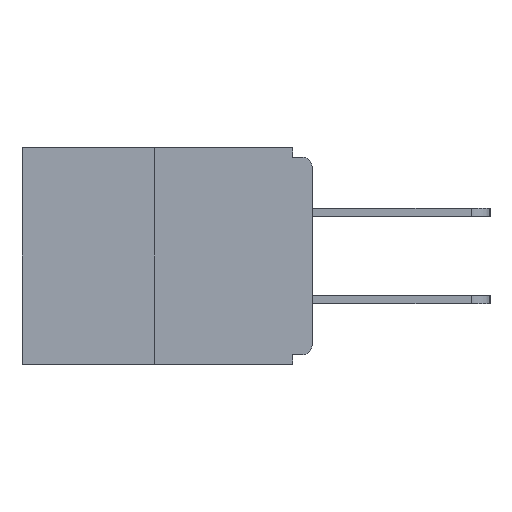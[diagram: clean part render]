
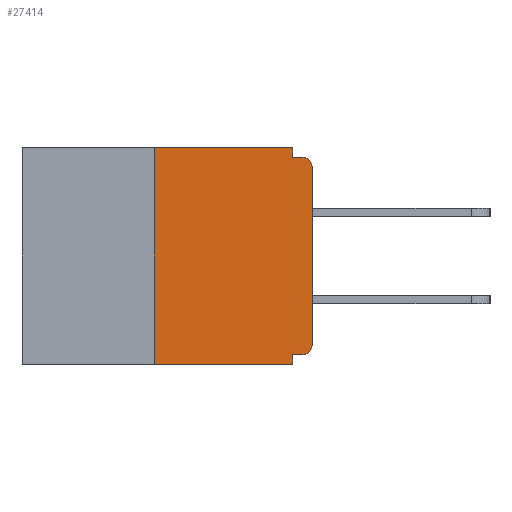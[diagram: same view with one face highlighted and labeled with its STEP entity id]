
A CAD part, left-side view. The second image highlights one B-rep face of the part: STEP entity #27414.
In plain terms, the highlighted planar face has unit normal (-1, 0, 0).
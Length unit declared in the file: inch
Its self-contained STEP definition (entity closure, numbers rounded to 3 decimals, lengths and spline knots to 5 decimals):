
#258 = VERTEX_POINT ( 'NONE', #12342 ) ;
#924 = CIRCLE ( 'NONE', #13292, 0.015 ) ;
#1094 = EDGE_CURVE ( 'NONE', #1641, #19054, #5235, .T. ) ;
#1258 = DIRECTION ( 'NONE',  ( 0., 0., -1. ) ) ;
#1621 = DIRECTION ( 'NONE',  ( 0., 0., -1. ) ) ;
#1641 = VERTEX_POINT ( 'NONE', #3744 ) ;
#2174 = DIRECTION ( 'NONE',  ( -1., 0., 0. ) ) ;
#2730 = CARTESIAN_POINT ( 'NONE',  ( 0., 0., -0.03 ) ) ;
#2752 = CARTESIAN_POINT ( 'NONE',  ( 0., 0.25, 0. ) ) ;
#3408 = ORIENTED_EDGE ( 'NONE', *, *, #23665, .F. ) ;
#3699 = EDGE_CURVE ( 'NONE', #7260, #28635, #924, .T. ) ;
#3744 = CARTESIAN_POINT ( 'NONE',  ( 0., 0.031, 0. ) ) ;
#3880 = ORIENTED_EDGE ( 'NONE', *, *, #10002, .F. ) ;
#4035 = DIRECTION ( 'NONE',  ( -1., 0., 0. ) ) ;
#4437 = VECTOR ( 'NONE', #1258, 39.37008 ) ;
#4613 = ORIENTED_EDGE ( 'NONE', *, *, #25031, .T. ) ;
#4737 = DIRECTION ( 'NONE',  ( 0., -1., 0. ) ) ;
#5190 = ORIENTED_EDGE ( 'NONE', *, *, #6835, .F. ) ;
#5235 = LINE ( 'NONE', #22909, #20057 ) ;
#6483 = CARTESIAN_POINT ( 'NONE',  ( 0., 0., -0.313 ) ) ;
#6586 = CARTESIAN_POINT ( 'NONE',  ( 0., 0., 0. ) ) ;
#6591 = EDGE_CURVE ( 'NONE', #25810, #1641, #14493, .T. ) ;
#6717 = LINE ( 'NONE', #6586, #25359 ) ;
#6772 = CARTESIAN_POINT ( 'NONE',  ( 0., 0., -0.328 ) ) ;
#6835 = EDGE_CURVE ( 'NONE', #19054, #28635, #21328, .T. ) ;
#7096 = VECTOR ( 'NONE', #27136, 39.37008 ) ;
#7260 = VERTEX_POINT ( 'NONE', #2730 ) ;
#8129 = CARTESIAN_POINT ( 'NONE',  ( 0., 0.46, -0.343 ) ) ;
#10002 = EDGE_CURVE ( 'NONE', #25297, #10109, #11707, .T. ) ;
#10061 = ORIENTED_EDGE ( 'NONE', *, *, #30148, .F. ) ;
#10109 = VERTEX_POINT ( 'NONE', #23777 ) ;
#10566 = ORIENTED_EDGE ( 'NONE', *, *, #18706, .T. ) ;
#11361 = VECTOR ( 'NONE', #28966, 39.37008 ) ;
#11636 = CARTESIAN_POINT ( 'NONE',  ( 0., 0.46, 0. ) ) ;
#11707 = LINE ( 'NONE', #18376, #4437 ) ;
#12342 = CARTESIAN_POINT ( 'NONE',  ( 0., 0.25, -0.343 ) ) ;
#13026 = DIRECTION ( 'NONE',  ( 0., -1., 0. ) ) ;
#13292 = AXIS2_PLACEMENT_3D ( 'NONE', #18622, #4035, #18407 ) ;
#13556 = DIRECTION ( 'NONE',  ( 0., 0., -1. ) ) ;
#13570 = LINE ( 'NONE', #2752, #7096 ) ;
#14385 = LINE ( 'NONE', #6772, #11361 ) ;
#14493 = LINE ( 'NONE', #27083, #30835 ) ;
#16056 = CARTESIAN_POINT ( 'NONE',  ( 0., 0.031, -0.328 ) ) ;
#16406 = CARTESIAN_POINT ( 'NONE',  ( 0., 0.25, 0. ) ) ;
#16729 = CARTESIAN_POINT ( 'NONE',  ( 0., 0.015, -0.015 ) ) ;
#17074 = DIRECTION ( 'NONE',  ( 0., -1., 0. ) ) ;
#18250 = EDGE_CURVE ( 'NONE', #18261, #7260, #6717, .T. ) ;
#18261 = VERTEX_POINT ( 'NONE', #6483 ) ;
#18376 = CARTESIAN_POINT ( 'NONE',  ( 0., 0.031, -0.343 ) ) ;
#18407 = DIRECTION ( 'NONE',  ( 0., 0., -1. ) ) ;
#18622 = CARTESIAN_POINT ( 'NONE',  ( 0., 0.015, -0.03 ) ) ;
#18706 = EDGE_CURVE ( 'NONE', #22608, #18261, #23068, .T. ) ;
#19008 = FACE_OUTER_BOUND ( 'NONE', #26814, .T. ) ;
#19054 = VERTEX_POINT ( 'NONE', #22838 ) ;
#19094 = CARTESIAN_POINT ( 'NONE',  ( 0., 0., -0.015 ) ) ;
#20057 = VECTOR ( 'NONE', #13556, 39.37008 ) ;
#20251 = ORIENTED_EDGE ( 'NONE', *, *, #1094, .F. ) ;
#20269 = AXIS2_PLACEMENT_3D ( 'NONE', #11636, #26398, #1621 ) ;
#21266 = PLANE ( 'NONE',  #20269 ) ;
#21328 = LINE ( 'NONE', #19094, #24752 ) ;
#21964 = ORIENTED_EDGE ( 'NONE', *, *, #18250, .T. ) ;
#22200 = VECTOR ( 'NONE', #13026, 39.37008 ) ;
#22608 = VERTEX_POINT ( 'NONE', #24995 ) ;
#22838 = CARTESIAN_POINT ( 'NONE',  ( 0., 0.031, -0.015 ) ) ;
#22909 = CARTESIAN_POINT ( 'NONE',  ( 0., 0.031, 0. ) ) ;
#23068 = CIRCLE ( 'NONE', #31440, 0.015 ) ;
#23607 = ORIENTED_EDGE ( 'NONE', *, *, #6591, .F. ) ;
#23665 = EDGE_CURVE ( 'NONE', #22608, #25297, #14385, .T. ) ;
#23777 = CARTESIAN_POINT ( 'NONE',  ( 0., 0.031, -0.343 ) ) ;
#24583 = ORIENTED_EDGE ( 'NONE', *, *, #3699, .T. ) ;
#24752 = VECTOR ( 'NONE', #4737, 39.37008 ) ;
#24995 = CARTESIAN_POINT ( 'NONE',  ( 0., 0.015, -0.328 ) ) ;
#25031 = EDGE_CURVE ( 'NONE', #258, #10109, #30561, .T. ) ;
#25297 = VERTEX_POINT ( 'NONE', #16056 ) ;
#25359 = VECTOR ( 'NONE', #30387, 39.37008 ) ;
#25810 = VERTEX_POINT ( 'NONE', #16406 ) ;
#26398 = DIRECTION ( 'NONE',  ( 1., 0., 0. ) ) ;
#26814 = EDGE_LOOP ( 'NONE', ( #23607, #10061, #4613, #3880, #3408, #10566, #21964, #24583, #5190, #20251 ) ) ;
#27083 = CARTESIAN_POINT ( 'NONE',  ( 0., 0.46, 0. ) ) ;
#27136 = DIRECTION ( 'NONE',  ( 0., 0., 1. ) ) ;
#27414 = ADVANCED_FACE ( 'NONE', ( #19008 ), #21266, .F. ) ;
#28635 = VERTEX_POINT ( 'NONE', #16729 ) ;
#28842 = DIRECTION ( 'NONE',  ( 0., 0., -1. ) ) ;
#28966 = DIRECTION ( 'NONE',  ( 0., 1., 0. ) ) ;
#30148 = EDGE_CURVE ( 'NONE', #258, #25810, #13570, .T. ) ;
#30387 = DIRECTION ( 'NONE',  ( 0., 0., 1. ) ) ;
#30561 = LINE ( 'NONE', #8129, #22200 ) ;
#30835 = VECTOR ( 'NONE', #17074, 39.37008 ) ;
#31396 = CARTESIAN_POINT ( 'NONE',  ( 0., 0.015, -0.313 ) ) ;
#31440 = AXIS2_PLACEMENT_3D ( 'NONE', #31396, #2174, #28842 ) ;
